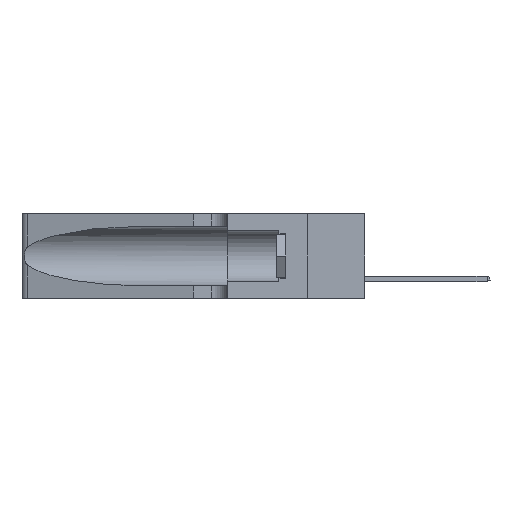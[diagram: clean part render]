
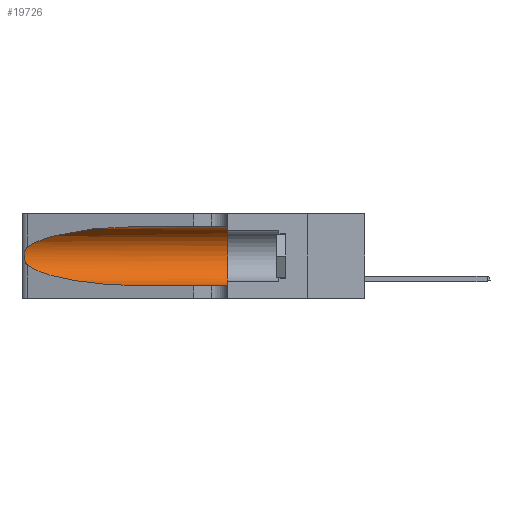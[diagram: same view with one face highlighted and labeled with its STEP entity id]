
A CAD part, left-side view. The second image highlights one B-rep face of the part: STEP entity #19726.
In plain terms, the highlighted cylindrical face has radius 3.308 mm (diameter 6.617 mm), a partial arc.
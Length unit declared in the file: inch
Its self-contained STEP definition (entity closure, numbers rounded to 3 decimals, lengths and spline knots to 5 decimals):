
#608 = CARTESIAN_POINT ( 'NONE',  ( 0.1305, 0.72297, 0.31525 ) ) ;
#1021 = CARTESIAN_POINT ( 'NONE',  ( 0.25854, 1.2359, 0.20912 ) ) ;
#1223 = ORIENTED_EDGE ( 'NONE', *, *, #7914, .F. ) ;
#1641 = CARTESIAN_POINT ( 'NONE',  ( 0.25639, 1.23186, 0.15144 ) ) ;
#1810 = VERTEX_POINT ( 'NONE', #24358 ) ;
#1999 = LINE ( 'NONE', #15137, #11821 ) ;
#2386 = EDGE_CURVE ( 'NONE', #2952, #28013, #1999, .T. ) ;
#2952 = VERTEX_POINT ( 'NONE', #18963 ) ;
#3306 = CARTESIAN_POINT ( 'NONE',  ( 0.25639, 1.23184, 0.21858 ) ) ;
#4132 = CARTESIAN_POINT ( 'NONE',  ( 0.1305, 0.35, 0.31525 ) ) ;
#5721 = CARTESIAN_POINT ( 'NONE',  ( 0.25856, 1.23593, 0.16098 ) ) ;
#5913 = B_SPLINE_CURVE_WITH_KNOTS ( 'NONE', 3,
 ( #24995, #17795, #3306, #13032, #1021, #11245, #10494, #25852, #17794, #5721, #13671, #1641, #8181, #13143 ),
 .UNSPECIFIED., .F., .F.,
 ( 4, 2, 2, 2, 2, 2, 4 ),
 ( 0., 0.00027, 0.00053, 0.00107, 0.0016, 0.00187, 0.00214 ),
 .UNSPECIFIED. ) ;
#7294 = DIRECTION ( 'NONE',  ( 0., 0., 1. ) ) ;
#7443 = CARTESIAN_POINT ( 'NONE',  ( 0.1305, 0.72297, 0.31525 ) ) ;
#7669 = CARTESIAN_POINT ( 'NONE',  ( 0.1305, 1.61858, 0.31525 ) ) ;
#7782 = VECTOR ( 'NONE', #14979, 39.37008 ) ;
#7791 = ORIENTED_EDGE ( 'NONE', *, *, #21035, .T. ) ;
#7819 = CARTESIAN_POINT ( 'NONE',  ( 0.1305, 0.35, 0.05475 ) ) ;
#7850 =( BOUNDED_CURVE ( )  B_SPLINE_CURVE ( 3, ( #21013, #11058, #20795, #16026 ),
 .UNSPECIFIED., .F., .T. ) 
 B_SPLINE_CURVE_WITH_KNOTS ( ( 4, 4 ),
 ( 3.44316, 4.71239 ),
 .UNSPECIFIED. ) 
 CURVE ( )  GEOMETRIC_REPRESENTATION_ITEM ( )  RATIONAL_B_SPLINE_CURVE ( ( 1., 0.87, 0.87, 1. ) ) 
 REPRESENTATION_ITEM ( '' )  );
#7914 = EDGE_CURVE ( 'NONE', #26894, #8399, #13093, .T. ) ;
#8181 = CARTESIAN_POINT ( 'NONE',  ( 0.25555, 1.22993, 0.14849 ) ) ;
#8244 =( BOUNDED_CURVE ( )  B_SPLINE_CURVE ( 3, ( #608, #29863, #10301, #24688 ),
 .UNSPECIFIED., .F., .T. ) 
 B_SPLINE_CURVE_WITH_KNOTS ( ( 4, 4 ),
 ( 1.5708, 2.84003 ),
 .UNSPECIFIED. ) 
 CURVE ( )  GEOMETRIC_REPRESENTATION_ITEM ( )  RATIONAL_B_SPLINE_CURVE ( ( 1., 0.87, 0.87, 1. ) ) 
 REPRESENTATION_ITEM ( '' )  );
#8399 = VERTEX_POINT ( 'NONE', #4132 ) ;
#8494 = CARTESIAN_POINT ( 'NONE',  ( 0.1305, 1.61858, 0.185 ) ) ;
#8593 = EDGE_CURVE ( 'NONE', #1810, #15313, #5913, .T. ) ;
#8678 = EDGE_LOOP ( 'NONE', ( #17797, #10364, #7791, #19755, #26822, #1223 ) ) ;
#8930 = AXIS2_PLACEMENT_3D ( 'NONE', #8494, #13351, #30179 ) ;
#10301 = CARTESIAN_POINT ( 'NONE',  ( 0.2373, 1.15595, 0.28018 ) ) ;
#10364 = ORIENTED_EDGE ( 'NONE', *, *, #8593, .T. ) ;
#10494 = CARTESIAN_POINT ( 'NONE',  ( 0.26075, 1.23896, 0.19203 ) ) ;
#11058 = CARTESIAN_POINT ( 'NONE',  ( 0.2373, 1.15595, 0.08982 ) ) ;
#11245 = CARTESIAN_POINT ( 'NONE',  ( 0.26018, 1.23835, 0.19895 ) ) ;
#11821 = VECTOR ( 'NONE', #17257, 39.37008 ) ;
#12083 = CIRCLE ( 'NONE', #30342, 0.13025 ) ;
#13032 = CARTESIAN_POINT ( 'NONE',  ( 0.25787, 1.23484, 0.2124 ) ) ;
#13093 = LINE ( 'NONE', #7669, #7782 ) ;
#13143 = CARTESIAN_POINT ( 'NONE',  ( 0.25487, 1.22718, 0.14631 ) ) ;
#13351 = DIRECTION ( 'NONE',  ( 0., -1., 0. ) ) ;
#13671 = CARTESIAN_POINT ( 'NONE',  ( 0.25789, 1.23486, 0.15765 ) ) ;
#14404 = CARTESIAN_POINT ( 'NONE',  ( 0.25487, 1.22718, 0.14631 ) ) ;
#14979 = DIRECTION ( 'NONE',  ( 0., -1., 0. ) ) ;
#15137 = CARTESIAN_POINT ( 'NONE',  ( 0.1305, 1.61858, 0.05475 ) ) ;
#15313 = VERTEX_POINT ( 'NONE', #14404 ) ;
#15835 = EDGE_CURVE ( 'NONE', #8399, #28013, #12083, .T. ) ;
#16026 = CARTESIAN_POINT ( 'NONE',  ( 0.1305, 0.72297, 0.05475 ) ) ;
#16532 = DIRECTION ( 'NONE',  ( 0., 1., 0. ) ) ;
#17119 = FACE_OUTER_BOUND ( 'NONE', #8678, .T. ) ;
#17257 = DIRECTION ( 'NONE',  ( 0., -1., 0. ) ) ;
#17794 = CARTESIAN_POINT ( 'NONE',  ( 0.26017, 1.23833, 0.17102 ) ) ;
#17795 = CARTESIAN_POINT ( 'NONE',  ( 0.25555, 1.22994, 0.2215 ) ) ;
#17797 = ORIENTED_EDGE ( 'NONE', *, *, #26950, .T. ) ;
#18963 = CARTESIAN_POINT ( 'NONE',  ( 0.1305, 0.72297, 0.05475 ) ) ;
#19726 = ADVANCED_FACE ( 'NONE', ( #17119 ), #22037, .F. ) ;
#19755 = ORIENTED_EDGE ( 'NONE', *, *, #2386, .T. ) ;
#20795 = CARTESIAN_POINT ( 'NONE',  ( 0.18966, 0.96281, 0.05475 ) ) ;
#21013 = CARTESIAN_POINT ( 'NONE',  ( 0.25487, 1.22718, 0.14631 ) ) ;
#21035 = EDGE_CURVE ( 'NONE', #15313, #2952, #7850, .T. ) ;
#22037 = CYLINDRICAL_SURFACE ( 'NONE', #8930, 0.13025 ) ;
#24358 = CARTESIAN_POINT ( 'NONE',  ( 0.25487, 1.22718, 0.22369 ) ) ;
#24688 = CARTESIAN_POINT ( 'NONE',  ( 0.25487, 1.22718, 0.22369 ) ) ;
#24995 = CARTESIAN_POINT ( 'NONE',  ( 0.25487, 1.22718, 0.22369 ) ) ;
#25852 = CARTESIAN_POINT ( 'NONE',  ( 0.26075, 1.23896, 0.178 ) ) ;
#26822 = ORIENTED_EDGE ( 'NONE', *, *, #15835, .F. ) ;
#26894 = VERTEX_POINT ( 'NONE', #7443 ) ;
#26950 = EDGE_CURVE ( 'NONE', #26894, #1810, #8244, .T. ) ;
#28013 = VERTEX_POINT ( 'NONE', #7819 ) ;
#29863 = CARTESIAN_POINT ( 'NONE',  ( 0.18966, 0.96281, 0.31525 ) ) ;
#30179 = DIRECTION ( 'NONE',  ( 0., 0., -1. ) ) ;
#30342 = AXIS2_PLACEMENT_3D ( 'NONE', #31013, #16532, #7294 ) ;
#31013 = CARTESIAN_POINT ( 'NONE',  ( 0.1305, 0.35, 0.185 ) ) ;
